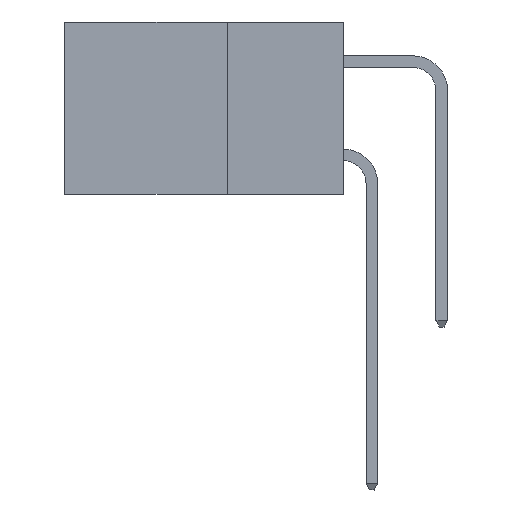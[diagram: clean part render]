
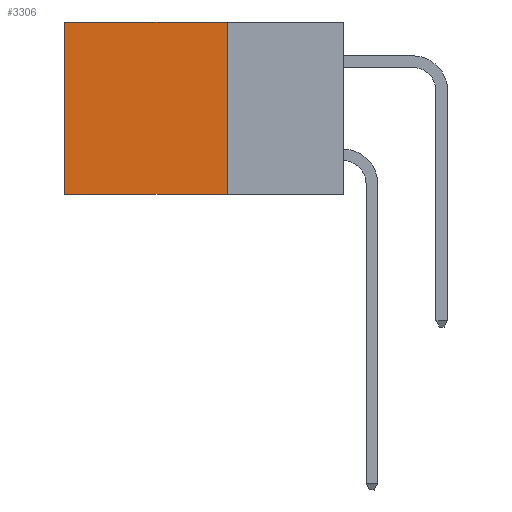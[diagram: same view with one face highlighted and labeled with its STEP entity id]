
A CAD part, left-side view. The second image highlights one B-rep face of the part: STEP entity #3306.
In plain terms, the highlighted planar face has unit normal (-1, 0, 0).
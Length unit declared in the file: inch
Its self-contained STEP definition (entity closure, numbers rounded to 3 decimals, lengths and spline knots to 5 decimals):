
#288 = CARTESIAN_POINT ( 'NONE',  ( 0.298, 0.25, -0.37 ) ) ;
#458 = CARTESIAN_POINT ( 'NONE',  ( 0.298, 0.25, -0.37 ) ) ;
#581 = VECTOR ( 'NONE', #1780, 39.37008 ) ;
#609 = CARTESIAN_POINT ( 'NONE',  ( 0.298, 0.25, 0. ) ) ;
#662 = VECTOR ( 'NONE', #4058, 39.37008 ) ;
#1072 = ORIENTED_EDGE ( 'NONE', *, *, #2222, .T. ) ;
#1780 = DIRECTION ( 'NONE',  ( 0., 0., -1. ) ) ;
#2069 = CARTESIAN_POINT ( 'NONE',  ( 0.298, 0.6, 0. ) ) ;
#2222 = EDGE_CURVE ( 'NONE', #10732, #9195, #9421, .T. ) ;
#2688 = DIRECTION ( 'NONE',  ( 0., 0., -1. ) ) ;
#3118 = VERTEX_POINT ( 'NONE', #458 ) ;
#3217 = EDGE_CURVE ( 'NONE', #9195, #10945, #5117, .T. ) ;
#3306 = ADVANCED_FACE ( 'NONE', ( #8049 ), #6930, .F. ) ;
#4058 = DIRECTION ( 'NONE',  ( 0., 1., 0. ) ) ;
#4084 = CARTESIAN_POINT ( 'NONE',  ( 0.298, 0.6, -0.37 ) ) ;
#4938 = VECTOR ( 'NONE', #8565, 39.37008 ) ;
#4981 = EDGE_LOOP ( 'NONE', ( #9011, #8367, #5169, #1072 ) ) ;
#5117 = LINE ( 'NONE', #2069, #4938 ) ;
#5169 = ORIENTED_EDGE ( 'NONE', *, *, #7661, .F. ) ;
#5907 = DIRECTION ( 'NONE',  ( 1., 0., 0. ) ) ;
#6930 = PLANE ( 'NONE',  #7345 ) ;
#7345 = AXIS2_PLACEMENT_3D ( 'NONE', #13586, #5907, #2688 ) ;
#7399 = CARTESIAN_POINT ( 'NONE',  ( 0.298, 0.6, 0. ) ) ;
#7661 = EDGE_CURVE ( 'NONE', #10732, #3118, #13155, .T. ) ;
#8049 = FACE_OUTER_BOUND ( 'NONE', #4981, .T. ) ;
#8367 = ORIENTED_EDGE ( 'NONE', *, *, #11359, .F. ) ;
#8565 = DIRECTION ( 'NONE',  ( 0., 0., -1. ) ) ;
#8741 = LINE ( 'NONE', #288, #9916 ) ;
#9011 = ORIENTED_EDGE ( 'NONE', *, *, #3217, .T. ) ;
#9195 = VERTEX_POINT ( 'NONE', #7399 ) ;
#9202 = DIRECTION ( 'NONE',  ( 0., 1., 0. ) ) ;
#9421 = LINE ( 'NONE', #11887, #662 ) ;
#9916 = VECTOR ( 'NONE', #9202, 39.37008 ) ;
#10732 = VERTEX_POINT ( 'NONE', #609 ) ;
#10945 = VERTEX_POINT ( 'NONE', #4084 ) ;
#11359 = EDGE_CURVE ( 'NONE', #3118, #10945, #8741, .T. ) ;
#11887 = CARTESIAN_POINT ( 'NONE',  ( 0.298, 0.25, 0. ) ) ;
#12827 = CARTESIAN_POINT ( 'NONE',  ( 0.298, 0.25, 0. ) ) ;
#13155 = LINE ( 'NONE', #12827, #581 ) ;
#13586 = CARTESIAN_POINT ( 'NONE',  ( 0.298, 0.25, 0. ) ) ;
